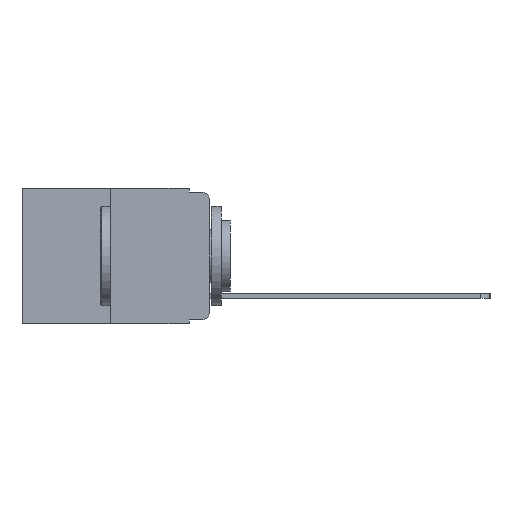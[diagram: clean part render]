
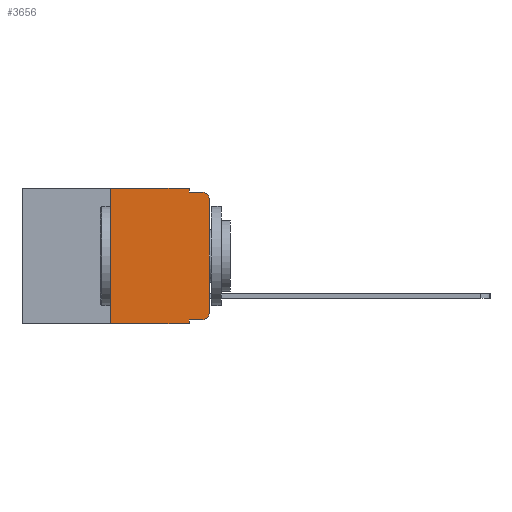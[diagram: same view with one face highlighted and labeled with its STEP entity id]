
A CAD part, left-side view. The second image highlights one B-rep face of the part: STEP entity #3656.
In plain terms, the highlighted planar face has unit normal (-1, 0, 0).
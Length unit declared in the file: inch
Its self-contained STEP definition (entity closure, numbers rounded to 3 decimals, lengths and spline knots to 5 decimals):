
#28 = DIRECTION ( 'NONE',  ( 0., 0., -1. ) ) ;
#226 = ORIENTED_EDGE ( 'NONE', *, *, #7582, .F. ) ;
#233 = DIRECTION ( 'NONE',  ( -1., 0., 0. ) ) ;
#344 = CARTESIAN_POINT ( 'NONE',  ( 0., 0.25, 0. ) ) ;
#358 = CARTESIAN_POINT ( 'NONE',  ( 0., 0., -0.03 ) ) ;
#382 = PLANE ( 'NONE',  #4444 ) ;
#454 = ORIENTED_EDGE ( 'NONE', *, *, #1703, .T. ) ;
#1013 = LINE ( 'NONE', #344, #6242 ) ;
#1075 = ORIENTED_EDGE ( 'NONE', *, *, #8325, .F. ) ;
#1225 = LINE ( 'NONE', #7271, #6418 ) ;
#1309 = CARTESIAN_POINT ( 'NONE',  ( 0., 0., -0.313 ) ) ;
#1315 = ORIENTED_EDGE ( 'NONE', *, *, #12009, .T. ) ;
#1465 = DIRECTION ( 'NONE',  ( 0., 0., 1. ) ) ;
#1572 = DIRECTION ( 'NONE',  ( 0., -1., 0. ) ) ;
#1588 = VERTEX_POINT ( 'NONE', #10705 ) ;
#1604 = FACE_OUTER_BOUND ( 'NONE', #5067, .T. ) ;
#1703 = EDGE_CURVE ( 'NONE', #7173, #9985, #1800, .T. ) ;
#1800 = LINE ( 'NONE', #10301, #9258 ) ;
#2058 = VERTEX_POINT ( 'NONE', #4411 ) ;
#2113 = ORIENTED_EDGE ( 'NONE', *, *, #8425, .T. ) ;
#2279 = ORIENTED_EDGE ( 'NONE', *, *, #2675, .T. ) ;
#2499 = VERTEX_POINT ( 'NONE', #1309 ) ;
#2642 = CARTESIAN_POINT ( 'NONE',  ( 0., 0.473, -0.343 ) ) ;
#2675 = EDGE_CURVE ( 'NONE', #2499, #7496, #11916, .T. ) ;
#2986 = ORIENTED_EDGE ( 'NONE', *, *, #4375, .T. ) ;
#3341 = ORIENTED_EDGE ( 'NONE', *, *, #4311, .F. ) ;
#3464 = CARTESIAN_POINT ( 'NONE',  ( 0., 0.25, 0. ) ) ;
#3583 = VERTEX_POINT ( 'NONE', #3464 ) ;
#3656 = ADVANCED_FACE ( 'NONE', ( #1604 ), #382, .F. ) ;
#4178 = VECTOR ( 'NONE', #11372, 39.37008 ) ;
#4311 = EDGE_CURVE ( 'NONE', #2058, #11100, #1225, .T. ) ;
#4375 = EDGE_CURVE ( 'NONE', #7496, #11100, #5526, .T. ) ;
#4411 = CARTESIAN_POINT ( 'NONE',  ( 0., 0.051, -0.01 ) ) ;
#4444 = AXIS2_PLACEMENT_3D ( 'NONE', #6629, #4461, #7237 ) ;
#4461 = DIRECTION ( 'NONE',  ( 1., 0., 0. ) ) ;
#4599 = ORIENTED_EDGE ( 'NONE', *, *, #11796, .F. ) ;
#4798 = ORIENTED_EDGE ( 'NONE', *, *, #5898, .F. ) ;
#5067 = EDGE_LOOP ( 'NONE', ( #2279, #2986, #3341, #4599, #226, #1075, #2113, #4798, #454, #1315 ) ) ;
#5526 = CIRCLE ( 'NONE', #7341, 0.02 ) ;
#5712 = CARTESIAN_POINT ( 'NONE',  ( 0., 0.051, 0. ) ) ;
#5898 = EDGE_CURVE ( 'NONE', #7173, #1588, #8814, .T. ) ;
#6116 = LINE ( 'NONE', #9358, #10559 ) ;
#6123 = CARTESIAN_POINT ( 'NONE',  ( 0., 0.051, -0.333 ) ) ;
#6242 = VECTOR ( 'NONE', #1465, 39.37008 ) ;
#6325 = DIRECTION ( 'NONE',  ( 0., 0., 1. ) ) ;
#6334 = DIRECTION ( 'NONE',  ( -1., 0., 0. ) ) ;
#6346 = DIRECTION ( 'NONE',  ( 0., -1., 0. ) ) ;
#6418 = VECTOR ( 'NONE', #6346, 39.37008 ) ;
#6451 = CARTESIAN_POINT ( 'NONE',  ( 0., 0., 0. ) ) ;
#6465 = DIRECTION ( 'NONE',  ( 0., 0., -1. ) ) ;
#6512 = CARTESIAN_POINT ( 'NONE',  ( 0., 0.02, -0.03 ) ) ;
#6629 = CARTESIAN_POINT ( 'NONE',  ( 0., 0.473, 0. ) ) ;
#7173 = VERTEX_POINT ( 'NONE', #6123 ) ;
#7237 = DIRECTION ( 'NONE',  ( 0., 0., -1. ) ) ;
#7271 = CARTESIAN_POINT ( 'NONE',  ( 0., 0.051, -0.01 ) ) ;
#7341 = AXIS2_PLACEMENT_3D ( 'NONE', #6512, #233, #7425 ) ;
#7425 = DIRECTION ( 'NONE',  ( 0., 0., -1. ) ) ;
#7496 = VERTEX_POINT ( 'NONE', #358 ) ;
#7521 = VERTEX_POINT ( 'NONE', #5712 ) ;
#7582 = EDGE_CURVE ( 'NONE', #3583, #7521, #6116, .T. ) ;
#7946 = VERTEX_POINT ( 'NONE', #12273 ) ;
#8241 = CARTESIAN_POINT ( 'NONE',  ( 0., 0.051, 0. ) ) ;
#8267 = VECTOR ( 'NONE', #6465, 39.37008 ) ;
#8325 = EDGE_CURVE ( 'NONE', #7946, #3583, #1013, .T. ) ;
#8425 = EDGE_CURVE ( 'NONE', #7946, #1588, #12277, .T. ) ;
#8814 = LINE ( 'NONE', #8241, #8267 ) ;
#9258 = VECTOR ( 'NONE', #11298, 39.37008 ) ;
#9358 = CARTESIAN_POINT ( 'NONE',  ( 0., 0.473, 0. ) ) ;
#9364 = VECTOR ( 'NONE', #6325, 39.37008 ) ;
#9985 = VERTEX_POINT ( 'NONE', #11799 ) ;
#10008 = VECTOR ( 'NONE', #1572, 39.37008 ) ;
#10301 = CARTESIAN_POINT ( 'NONE',  ( 0., 0.051, -0.333 ) ) ;
#10523 = CARTESIAN_POINT ( 'NONE',  ( 0., 0.051, 0. ) ) ;
#10559 = VECTOR ( 'NONE', #11945, 39.37008 ) ;
#10705 = CARTESIAN_POINT ( 'NONE',  ( 0., 0.051, -0.343 ) ) ;
#10975 = AXIS2_PLACEMENT_3D ( 'NONE', #11592, #6334, #28 ) ;
#11100 = VERTEX_POINT ( 'NONE', #11530 ) ;
#11160 = LINE ( 'NONE', #10523, #4178 ) ;
#11298 = DIRECTION ( 'NONE',  ( 0., -1., 0. ) ) ;
#11372 = DIRECTION ( 'NONE',  ( 0., 0., -1. ) ) ;
#11530 = CARTESIAN_POINT ( 'NONE',  ( 0., 0.02, -0.01 ) ) ;
#11592 = CARTESIAN_POINT ( 'NONE',  ( 0., 0.02, -0.313 ) ) ;
#11796 = EDGE_CURVE ( 'NONE', #7521, #2058, #11160, .T. ) ;
#11799 = CARTESIAN_POINT ( 'NONE',  ( 0., 0.02, -0.333 ) ) ;
#11810 = CIRCLE ( 'NONE', #10975, 0.02 ) ;
#11916 = LINE ( 'NONE', #6451, #9364 ) ;
#11945 = DIRECTION ( 'NONE',  ( 0., -1., 0. ) ) ;
#12009 = EDGE_CURVE ( 'NONE', #9985, #2499, #11810, .T. ) ;
#12273 = CARTESIAN_POINT ( 'NONE',  ( 0., 0.25, -0.343 ) ) ;
#12277 = LINE ( 'NONE', #2642, #10008 ) ;
